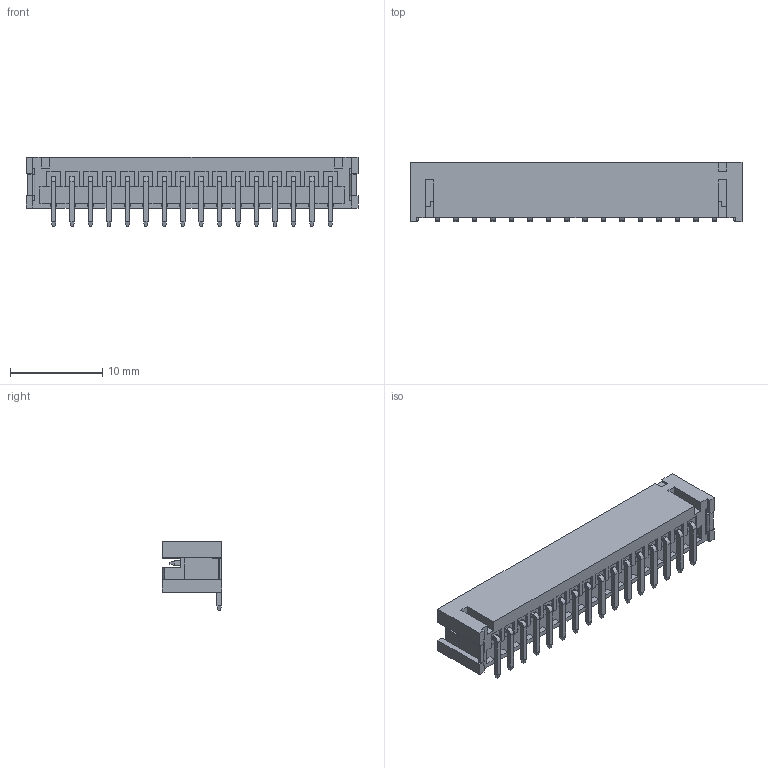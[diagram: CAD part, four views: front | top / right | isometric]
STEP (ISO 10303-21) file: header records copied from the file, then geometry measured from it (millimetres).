
FILE_DESCRIPTION (( 'STEP AP203' ), '1' );
FILE_NAME ('140-516-417-011.STEP', '2020-03-31T20:08:38', ( '' ), ( '' ), 'SwSTEP 2.0', 'SolidWorks 2016', '' );
FILE_SCHEMA (( 'CONFIG_CONTROL_DESIGN' ));
Length unit declared in the file: millimetre
Products named in the file (4): V SMT Housing_516; 140-516-417-011; V SMT Contact; V SMT Pad
Assembly tree (19 placements, depth 2):
  140-516-417-011
    V SMT Housing_516
    V SMT Contact  x16
    V SMT Pad  x2
Bounding box: 36 x 6.4 x 7.5 mm (x, y, z)
Volume: 506.1 mm3; surface area: 1837.9 mm2
Topology: 19 solids, 19 shells, 708 faces, 1756 edges, 1082 vertices
Faces by surface type: plane 672, cylinder 36
Entity records: 12742 total; most frequent: CARTESIAN_POINT 2144, ORIENTED_EDGE 2120, DIRECTION 1840, EDGE_CURVE 1060, VECTOR 1052, LINE 1052, VERTEX_POINT 698, EDGE_LOOP 396
